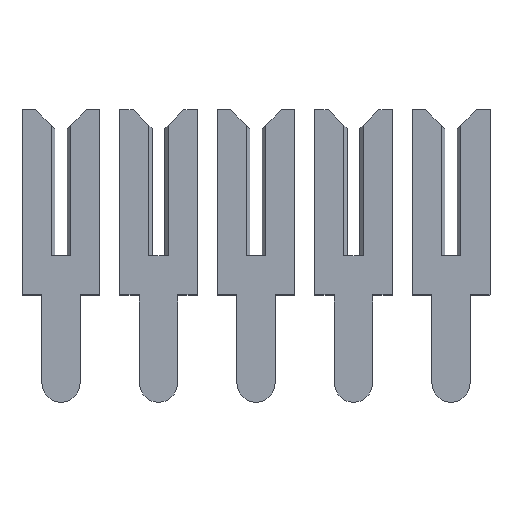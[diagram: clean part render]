
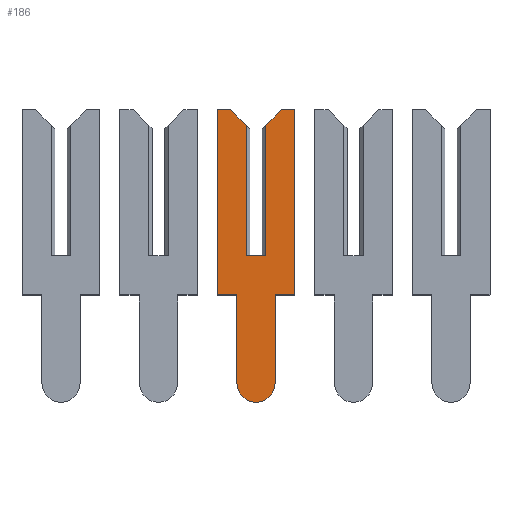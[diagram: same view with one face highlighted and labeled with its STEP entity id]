
A CAD part, top view. The second image highlights one B-rep face of the part: STEP entity #186.
In plain terms, the highlighted face is planar.
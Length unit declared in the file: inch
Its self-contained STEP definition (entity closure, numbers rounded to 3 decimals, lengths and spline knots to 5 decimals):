
#7 = EDGE_CURVE ( 'NONE', #572, #648, #851, .T. ) ;
#13 = VECTOR ( 'NONE', #428, 39.37008 ) ;
#20 = CARTESIAN_POINT ( 'NONE',  ( -0.01, 0., 0.01 ) ) ;
#26 = ORIENTED_EDGE ( 'NONE', *, *, #195, .F. ) ;
#29 = EDGE_CURVE ( 'NONE', #104, #873, #687, .T. ) ;
#30 = EDGE_CURVE ( 'NONE', #241, #515, #134, .T. ) ;
#41 = CARTESIAN_POINT ( 'NONE',  ( -0.01, 0.15, 0.026 ) ) ;
#82 = VECTOR ( 'NONE', #458, 39.37008 ) ;
#83 = LINE ( 'NONE', #439, #826 ) ;
#85 = ORIENTED_EDGE ( 'NONE', *, *, #906, .F. ) ;
#87 = CARTESIAN_POINT ( 'NONE',  ( -0.01, -0.04, 0.04 ) ) ;
#100 = CARTESIAN_POINT ( 'NONE',  ( -0.01, -0.1305, 0. ) ) ;
#104 = VERTEX_POINT ( 'NONE', #957 ) ;
#105 = CARTESIAN_POINT ( 'NONE',  ( -0.01, 0.15, 0.04 ) ) ;
#108 = CARTESIAN_POINT ( 'NONE',  ( -0.01, -0.1305, -0.0195 ) ) ;
#109 = AXIS2_PLACEMENT_3D ( 'NONE', #382, #149, #672 ) ;
#112 = CARTESIAN_POINT ( 'NONE',  ( -0.01, -0.04, -0.0195 ) ) ;
#114 = CARTESIAN_POINT ( 'NONE',  ( -0.01, -0.1305, 0.0195 ) ) ;
#117 = CARTESIAN_POINT ( 'NONE',  ( -0.01, 0., 0.0065 ) ) ;
#119 = VECTOR ( 'NONE', #498, 39.37008 ) ;
#121 = DIRECTION ( 'NONE',  ( 0., 0., 1. ) ) ;
#134 = LINE ( 'NONE', #117, #635 ) ;
#149 = DIRECTION ( 'NONE',  ( 1., 0., 0. ) ) ;
#174 = CARTESIAN_POINT ( 'NONE',  ( -0.01, 0.15, 0.01 ) ) ;
#179 = ORIENTED_EDGE ( 'NONE', *, *, #839, .F. ) ;
#185 = CARTESIAN_POINT ( 'NONE',  ( -0.01, -0.04, -0.04 ) ) ;
#186 = ADVANCED_FACE ( 'NONE', ( #260 ), #304, .F. ) ;
#192 = CARTESIAN_POINT ( 'NONE',  ( -0.01, 0.1305, 0.0065 ) ) ;
#195 = EDGE_CURVE ( 'NONE', #873, #912, #83, .T. ) ;
#199 = CARTESIAN_POINT ( 'NONE',  ( -0.01, -0.04, 0.0195 ) ) ;
#200 = LINE ( 'NONE', #557, #286 ) ;
#221 = ORIENTED_EDGE ( 'NONE', *, *, #29, .F. ) ;
#230 = EDGE_LOOP ( 'NONE', ( #636, #885, #773, #431, #634, #626, #179, #690, #874, #85, #502, #26, #221, #582 ) ) ;
#241 = VERTEX_POINT ( 'NONE', #370 ) ;
#260 = FACE_OUTER_BOUND ( 'NONE', #230, .T. ) ;
#262 = DIRECTION ( 'NONE',  ( 0., 1., 0. ) ) ;
#270 = VECTOR ( 'NONE', #846, 39.37008 ) ;
#273 = DIRECTION ( 'NONE',  ( 0., 0., 1. ) ) ;
#286 = VECTOR ( 'NONE', #915, 39.37008 ) ;
#299 = EDGE_CURVE ( 'NONE', #912, #942, #487, .T. ) ;
#304 = PLANE ( 'NONE',  #109 ) ;
#343 = DIRECTION ( 'NONE',  ( 0., 0., -1. ) ) ;
#353 = VERTEX_POINT ( 'NONE', #764 ) ;
#370 = CARTESIAN_POINT ( 'NONE',  ( -0.01, 0., -0.01 ) ) ;
#382 = CARTESIAN_POINT ( 'NONE',  ( -0.01, -0.1305, 0. ) ) ;
#401 = CARTESIAN_POINT ( 'NONE',  ( -0.01, 0.134, 0.01 ) ) ;
#415 = LINE ( 'NONE', #174, #782 ) ;
#416 = LINE ( 'NONE', #192, #270 ) ;
#422 = CARTESIAN_POINT ( 'NONE',  ( -0.01, 0.15, -0.026 ) ) ;
#428 = DIRECTION ( 'NONE',  ( 0., 0., 1. ) ) ;
#431 = ORIENTED_EDGE ( 'NONE', *, *, #556, .F. ) ;
#439 = CARTESIAN_POINT ( 'NONE',  ( -0.01, 0.15, 0.04 ) ) ;
#458 = DIRECTION ( 'NONE',  ( 0., 0., -1. ) ) ;
#482 = DIRECTION ( 'NONE',  ( 0., -1., 0. ) ) ;
#487 = LINE ( 'NONE', #87, #82 ) ;
#498 = DIRECTION ( 'NONE',  ( 0., 1., 0. ) ) ;
#501 = CARTESIAN_POINT ( 'NONE',  ( -0.01, 0.15, -0.04 ) ) ;
#502 = ORIENTED_EDGE ( 'NONE', *, *, #299, .F. ) ;
#504 = EDGE_CURVE ( 'NONE', #837, #695, #631, .T. ) ;
#507 = VECTOR ( 'NONE', #853, 39.37008 ) ;
#515 = VERTEX_POINT ( 'NONE', #20 ) ;
#518 = VERTEX_POINT ( 'NONE', #770 ) ;
#539 = EDGE_CURVE ( 'NONE', #553, #515, #415, .T. ) ;
#553 = VERTEX_POINT ( 'NONE', #401 ) ;
#556 = EDGE_CURVE ( 'NONE', #648, #353, #200, .T. ) ;
#557 = CARTESIAN_POINT ( 'NONE',  ( -0.01, 0.1305, -0.0065 ) ) ;
#564 = VECTOR ( 'NONE', #343, 39.37008 ) ;
#565 = LINE ( 'NONE', #633, #587 ) ;
#570 = CARTESIAN_POINT ( 'NONE',  ( -0.01, -0.1305, -0.01 ) ) ;
#572 = VERTEX_POINT ( 'NONE', #698 ) ;
#576 = VECTOR ( 'NONE', #262, 39.37008 ) ;
#582 = ORIENTED_EDGE ( 'NONE', *, *, #682, .F. ) ;
#587 = VECTOR ( 'NONE', #715, 39.37008 ) ;
#591 = DIRECTION ( 'NONE',  ( 0., -1., 0. ) ) ;
#595 = VECTOR ( 'NONE', #273, 39.37008 ) ;
#626 = ORIENTED_EDGE ( 'NONE', *, *, #868, .F. ) ;
#631 = CIRCLE ( 'NONE', #724, 0.0195 ) ;
#633 = CARTESIAN_POINT ( 'NONE',  ( -0.01, -0.04, 0.0195 ) ) ;
#634 = ORIENTED_EDGE ( 'NONE', *, *, #7, .F. ) ;
#635 = VECTOR ( 'NONE', #121, 39.37008 ) ;
#636 = ORIENTED_EDGE ( 'NONE', *, *, #539, .T. ) ;
#648 = VERTEX_POINT ( 'NONE', #694 ) ;
#672 = DIRECTION ( 'NONE',  ( 0., 0., -1. ) ) ;
#677 = LINE ( 'NONE', #501, #576 ) ;
#682 = EDGE_CURVE ( 'NONE', #553, #104, #416, .T. ) ;
#687 = LINE ( 'NONE', #41, #13 ) ;
#690 = ORIENTED_EDGE ( 'NONE', *, *, #794, .F. ) ;
#694 = CARTESIAN_POINT ( 'NONE',  ( -0.01, 0.15, -0.026 ) ) ;
#695 = VERTEX_POINT ( 'NONE', #108 ) ;
#698 = CARTESIAN_POINT ( 'NONE',  ( -0.01, 0.15, -0.04 ) ) ;
#700 = LINE ( 'NONE', #570, #507 ) ;
#713 = LINE ( 'NONE', #112, #119 ) ;
#715 = DIRECTION ( 'NONE',  ( 0., -1., 0. ) ) ;
#724 = AXIS2_PLACEMENT_3D ( 'NONE', #100, #778, #836 ) ;
#744 = VERTEX_POINT ( 'NONE', #185 ) ;
#763 = LINE ( 'NONE', #854, #564 ) ;
#764 = CARTESIAN_POINT ( 'NONE',  ( -0.01, 0.134, -0.01 ) ) ;
#770 = CARTESIAN_POINT ( 'NONE',  ( -0.01, -0.04, -0.0195 ) ) ;
#773 = ORIENTED_EDGE ( 'NONE', *, *, #844, .F. ) ;
#778 = DIRECTION ( 'NONE',  ( 1., 0., 0. ) ) ;
#779 = CARTESIAN_POINT ( 'NONE',  ( -0.01, -0.04, 0.04 ) ) ;
#782 = VECTOR ( 'NONE', #482, 39.37008 ) ;
#794 = EDGE_CURVE ( 'NONE', #695, #518, #713, .T. ) ;
#826 = VECTOR ( 'NONE', #591, 39.37008 ) ;
#836 = DIRECTION ( 'NONE',  ( 0., 0., -1. ) ) ;
#837 = VERTEX_POINT ( 'NONE', #114 ) ;
#839 = EDGE_CURVE ( 'NONE', #518, #744, #763, .T. ) ;
#844 = EDGE_CURVE ( 'NONE', #353, #241, #700, .T. ) ;
#846 = DIRECTION ( 'NONE',  ( 0., 0.707, 0.707 ) ) ;
#851 = LINE ( 'NONE', #422, #595 ) ;
#853 = DIRECTION ( 'NONE',  ( 0., -1., 0. ) ) ;
#854 = CARTESIAN_POINT ( 'NONE',  ( -0.01, -0.04, -0.04 ) ) ;
#868 = EDGE_CURVE ( 'NONE', #744, #572, #677, .T. ) ;
#873 = VERTEX_POINT ( 'NONE', #105 ) ;
#874 = ORIENTED_EDGE ( 'NONE', *, *, #504, .F. ) ;
#885 = ORIENTED_EDGE ( 'NONE', *, *, #30, .F. ) ;
#906 = EDGE_CURVE ( 'NONE', #942, #837, #565, .T. ) ;
#912 = VERTEX_POINT ( 'NONE', #779 ) ;
#915 = DIRECTION ( 'NONE',  ( 0., -0.707, 0.707 ) ) ;
#942 = VERTEX_POINT ( 'NONE', #199 ) ;
#957 = CARTESIAN_POINT ( 'NONE',  ( -0.01, 0.15, 0.026 ) ) ;
